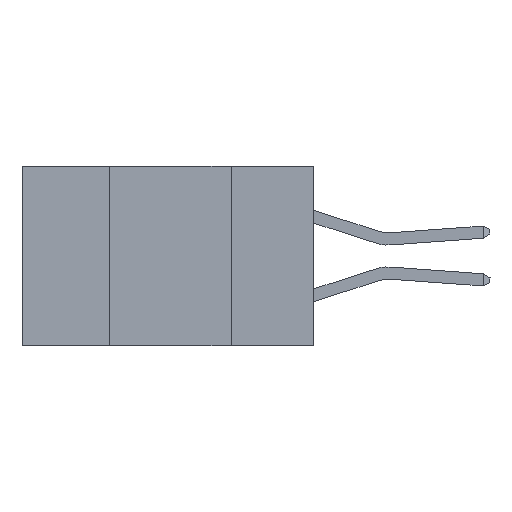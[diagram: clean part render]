
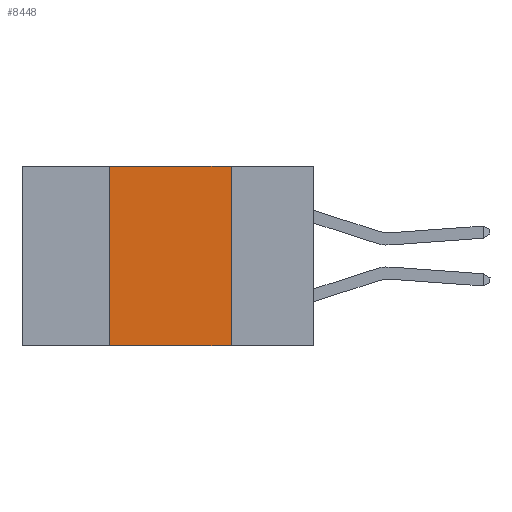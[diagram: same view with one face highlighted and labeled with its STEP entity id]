
A CAD part, left-side view. The second image highlights one B-rep face of the part: STEP entity #8448.
In plain terms, the highlighted planar face has unit normal (-1, 0, 0).
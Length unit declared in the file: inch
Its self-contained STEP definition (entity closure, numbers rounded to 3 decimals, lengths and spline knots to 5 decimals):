
#4 = DIRECTION ( 'NONE',  ( 0., -1., 0. ) ) ;
#248 = DIRECTION ( 'NONE',  ( 0., 0., -1. ) ) ;
#1664 = ORIENTED_EDGE ( 'NONE', *, *, #19886, .F. ) ;
#1897 = DIRECTION ( 'NONE',  ( 1., 0., 0. ) ) ;
#2443 = FACE_OUTER_BOUND ( 'NONE', #13534, .T. ) ;
#3557 = EDGE_CURVE ( 'NONE', #17481, #19165, #17510, .T. ) ;
#3830 = ORIENTED_EDGE ( 'NONE', *, *, #8658, .F. ) ;
#3954 = PLANE ( 'NONE',  #12487 ) ;
#4232 = DIRECTION ( 'NONE',  ( 0., 0., -1. ) ) ;
#4946 = LINE ( 'NONE', #7496, #21905 ) ;
#5059 = VECTOR ( 'NONE', #21600, 39.37008 ) ;
#5552 = LINE ( 'NONE', #22215, #19709 ) ;
#6176 = VECTOR ( 'NONE', #4, 39.37008 ) ;
#6290 = CARTESIAN_POINT ( 'NONE',  ( 0., 0.17, -0.37 ) ) ;
#7206 = LINE ( 'NONE', #13034, #6176 ) ;
#7496 = CARTESIAN_POINT ( 'NONE',  ( 0., 0.6, -0.37 ) ) ;
#8448 = ADVANCED_FACE ( 'NONE', ( #2443 ), #3954, .F. ) ;
#8658 = EDGE_CURVE ( 'NONE', #15134, #10936, #5552, .T. ) ;
#10936 = VERTEX_POINT ( 'NONE', #6290 ) ;
#12487 = AXIS2_PLACEMENT_3D ( 'NONE', #21835, #1897, #4232 ) ;
#13034 = CARTESIAN_POINT ( 'NONE',  ( 0., 0.6, 0. ) ) ;
#13534 = EDGE_LOOP ( 'NONE', ( #3830, #1664, #20369, #25476 ) ) ;
#14353 = DIRECTION ( 'NONE',  ( 0., -1., 0. ) ) ;
#15134 = VERTEX_POINT ( 'NONE', #25188 ) ;
#17180 = EDGE_CURVE ( 'NONE', #17481, #10936, #4946, .T. ) ;
#17439 = CARTESIAN_POINT ( 'NONE',  ( 0., 0.42, -0.37 ) ) ;
#17481 = VERTEX_POINT ( 'NONE', #17439 ) ;
#17510 = LINE ( 'NONE', #24095, #5059 ) ;
#19165 = VERTEX_POINT ( 'NONE', #24118 ) ;
#19709 = VECTOR ( 'NONE', #248, 39.37008 ) ;
#19886 = EDGE_CURVE ( 'NONE', #19165, #15134, #7206, .T. ) ;
#20369 = ORIENTED_EDGE ( 'NONE', *, *, #3557, .F. ) ;
#21600 = DIRECTION ( 'NONE',  ( 0., 0., 1. ) ) ;
#21835 = CARTESIAN_POINT ( 'NONE',  ( 0., 0.6, 0. ) ) ;
#21905 = VECTOR ( 'NONE', #14353, 39.37008 ) ;
#22215 = CARTESIAN_POINT ( 'NONE',  ( 0., 0.17, 0. ) ) ;
#24095 = CARTESIAN_POINT ( 'NONE',  ( 0., 0.42, 0. ) ) ;
#24118 = CARTESIAN_POINT ( 'NONE',  ( 0., 0.42, 0. ) ) ;
#25188 = CARTESIAN_POINT ( 'NONE',  ( 0., 0.17, 0. ) ) ;
#25476 = ORIENTED_EDGE ( 'NONE', *, *, #17180, .T. ) ;
